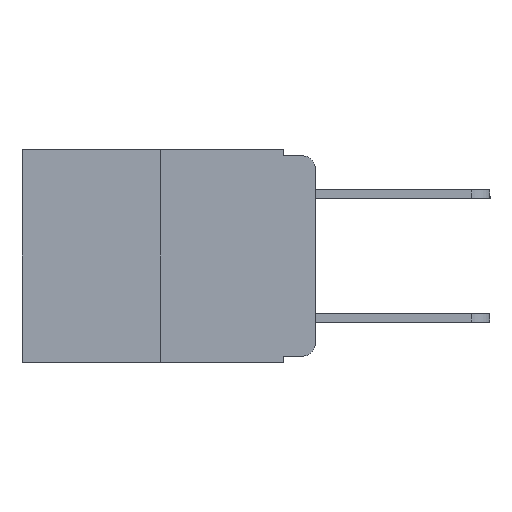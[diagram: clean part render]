
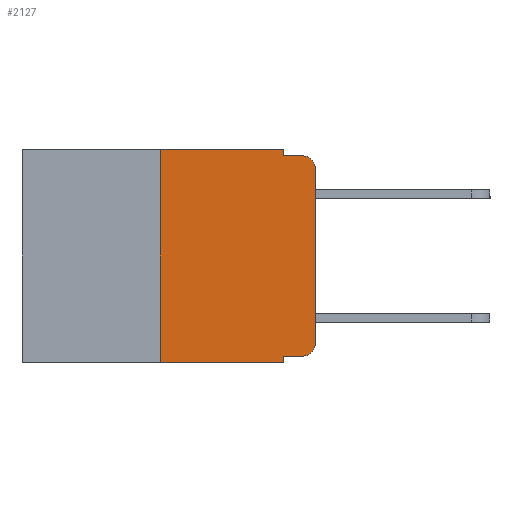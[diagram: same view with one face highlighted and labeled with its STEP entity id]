
A CAD part, left-side view. The second image highlights one B-rep face of the part: STEP entity #2127.
In plain terms, the highlighted planar face has unit normal (-1, 0, 0).
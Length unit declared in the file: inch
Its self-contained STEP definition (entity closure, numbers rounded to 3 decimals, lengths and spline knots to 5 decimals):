
#251 = CARTESIAN_POINT ( 'NONE',  ( 0., 0.02, -0.333 ) ) ;
#286 = DIRECTION ( 'NONE',  ( 0., 0., -1. ) ) ;
#292 = VECTOR ( 'NONE', #10526, 39.37008 ) ;
#388 = EDGE_LOOP ( 'NONE', ( #7040, #11678, #4794, #8635, #3206, #7563, #4962, #2960, #675, #3124 ) ) ;
#556 = CARTESIAN_POINT ( 'NONE',  ( 0., 0.051, 0. ) ) ;
#654 = VECTOR ( 'NONE', #4950, 39.37008 ) ;
#675 = ORIENTED_EDGE ( 'NONE', *, *, #6849, .T. ) ;
#803 = VERTEX_POINT ( 'NONE', #7510 ) ;
#924 = DIRECTION ( 'NONE',  ( 0., -1., 0. ) ) ;
#1088 = VERTEX_POINT ( 'NONE', #10537 ) ;
#1092 = DIRECTION ( 'NONE',  ( -1., 0., 0. ) ) ;
#1163 = FACE_OUTER_BOUND ( 'NONE', #388, .T. ) ;
#1445 = EDGE_CURVE ( 'NONE', #8519, #1088, #5009, .T. ) ;
#1622 = LINE ( 'NONE', #556, #292 ) ;
#1637 = LINE ( 'NONE', #4204, #3473 ) ;
#2127 = ADVANCED_FACE ( 'NONE', ( #1163 ), #10424, .F. ) ;
#2240 = EDGE_CURVE ( 'NONE', #9721, #8519, #1637, .T. ) ;
#2330 = VERTEX_POINT ( 'NONE', #251 ) ;
#2564 = VECTOR ( 'NONE', #924, 39.37008 ) ;
#2728 = CARTESIAN_POINT ( 'NONE',  ( 0., 0., -0.03 ) ) ;
#2746 = DIRECTION ( 'NONE',  ( 0., 0., 1. ) ) ;
#2827 = CARTESIAN_POINT ( 'NONE',  ( 0., 0.02, -0.03 ) ) ;
#2960 = ORIENTED_EDGE ( 'NONE', *, *, #11437, .F. ) ;
#3124 = ORIENTED_EDGE ( 'NONE', *, *, #10602, .T. ) ;
#3206 = ORIENTED_EDGE ( 'NONE', *, *, #1445, .F. ) ;
#3257 = DIRECTION ( 'NONE',  ( 1., 0., 0. ) ) ;
#3332 = VECTOR ( 'NONE', #8884, 39.37008 ) ;
#3473 = VECTOR ( 'NONE', #2746, 39.37008 ) ;
#3682 = AXIS2_PLACEMENT_3D ( 'NONE', #2827, #11299, #4958 ) ;
#3985 = EDGE_CURVE ( 'NONE', #10911, #7688, #11540, .T. ) ;
#4204 = CARTESIAN_POINT ( 'NONE',  ( 0., 0.25, 0. ) ) ;
#4368 = CARTESIAN_POINT ( 'NONE',  ( 0., 0.473, -0.343 ) ) ;
#4652 = CARTESIAN_POINT ( 'NONE',  ( 0., 0.25, 0. ) ) ;
#4794 = ORIENTED_EDGE ( 'NONE', *, *, #9701, .F. ) ;
#4950 = DIRECTION ( 'NONE',  ( 0., -1., 0. ) ) ;
#4958 = DIRECTION ( 'NONE',  ( 0., 0., -1. ) ) ;
#4962 = ORIENTED_EDGE ( 'NONE', *, *, #7101, .T. ) ;
#5009 = LINE ( 'NONE', #9514, #654 ) ;
#5138 = EDGE_CURVE ( 'NONE', #7688, #11702, #7276, .T. ) ;
#5379 = LINE ( 'NONE', #10775, #3332 ) ;
#5409 = VECTOR ( 'NONE', #7083, 39.37008 ) ;
#5524 = LINE ( 'NONE', #9967, #9989 ) ;
#5914 = CARTESIAN_POINT ( 'NONE',  ( 0., 0.473, 0. ) ) ;
#6209 = CARTESIAN_POINT ( 'NONE',  ( 0., 0.25, -0.343 ) ) ;
#6263 = LINE ( 'NONE', #10000, #2564 ) ;
#6674 = AXIS2_PLACEMENT_3D ( 'NONE', #5914, #3257, #286 ) ;
#6849 = EDGE_CURVE ( 'NONE', #803, #2330, #6263, .T. ) ;
#7033 = EDGE_CURVE ( 'NONE', #1088, #10306, #1622, .T. ) ;
#7040 = ORIENTED_EDGE ( 'NONE', *, *, #3985, .T. ) ;
#7083 = DIRECTION ( 'NONE',  ( 0., -1., 0. ) ) ;
#7101 = EDGE_CURVE ( 'NONE', #9721, #7293, #8863, .T. ) ;
#7108 = CIRCLE ( 'NONE', #9001, 0.02 ) ;
#7276 = CIRCLE ( 'NONE', #3682, 0.02 ) ;
#7293 = VERTEX_POINT ( 'NONE', #7424 ) ;
#7424 = CARTESIAN_POINT ( 'NONE',  ( 0., 0.051, -0.343 ) ) ;
#7510 = CARTESIAN_POINT ( 'NONE',  ( 0., 0.051, -0.333 ) ) ;
#7563 = ORIENTED_EDGE ( 'NONE', *, *, #2240, .F. ) ;
#7688 = VERTEX_POINT ( 'NONE', #2728 ) ;
#8026 = CARTESIAN_POINT ( 'NONE',  ( 0., 0., 0. ) ) ;
#8177 = DIRECTION ( 'NONE',  ( 0., 0., -1. ) ) ;
#8377 = DIRECTION ( 'NONE',  ( 0., 0., -1. ) ) ;
#8418 = CARTESIAN_POINT ( 'NONE',  ( 0., 0.051, -0.01 ) ) ;
#8519 = VERTEX_POINT ( 'NONE', #4652 ) ;
#8635 = ORIENTED_EDGE ( 'NONE', *, *, #7033, .F. ) ;
#8863 = LINE ( 'NONE', #4368, #5409 ) ;
#8884 = DIRECTION ( 'NONE',  ( 0., -1., 0. ) ) ;
#9001 = AXIS2_PLACEMENT_3D ( 'NONE', #9224, #1092, #8377 ) ;
#9052 = CARTESIAN_POINT ( 'NONE',  ( 0., 0.02, -0.01 ) ) ;
#9224 = CARTESIAN_POINT ( 'NONE',  ( 0., 0.02, -0.313 ) ) ;
#9514 = CARTESIAN_POINT ( 'NONE',  ( 0., 0.473, 0. ) ) ;
#9701 = EDGE_CURVE ( 'NONE', #10306, #11702, #5379, .T. ) ;
#9705 = DIRECTION ( 'NONE',  ( 0., 0., 1. ) ) ;
#9721 = VERTEX_POINT ( 'NONE', #6209 ) ;
#9967 = CARTESIAN_POINT ( 'NONE',  ( 0., 0.051, 0. ) ) ;
#9989 = VECTOR ( 'NONE', #8177, 39.37008 ) ;
#10000 = CARTESIAN_POINT ( 'NONE',  ( 0., 0.051, -0.333 ) ) ;
#10306 = VERTEX_POINT ( 'NONE', #8418 ) ;
#10424 = PLANE ( 'NONE',  #6674 ) ;
#10526 = DIRECTION ( 'NONE',  ( 0., 0., -1. ) ) ;
#10537 = CARTESIAN_POINT ( 'NONE',  ( 0., 0.051, 0. ) ) ;
#10581 = CARTESIAN_POINT ( 'NONE',  ( 0., 0., -0.313 ) ) ;
#10602 = EDGE_CURVE ( 'NONE', #2330, #10911, #7108, .T. ) ;
#10775 = CARTESIAN_POINT ( 'NONE',  ( 0., 0.051, -0.01 ) ) ;
#10911 = VERTEX_POINT ( 'NONE', #10581 ) ;
#11299 = DIRECTION ( 'NONE',  ( -1., 0., 0. ) ) ;
#11390 = VECTOR ( 'NONE', #9705, 39.37008 ) ;
#11437 = EDGE_CURVE ( 'NONE', #803, #7293, #5524, .T. ) ;
#11540 = LINE ( 'NONE', #8026, #11390 ) ;
#11678 = ORIENTED_EDGE ( 'NONE', *, *, #5138, .T. ) ;
#11702 = VERTEX_POINT ( 'NONE', #9052 ) ;
